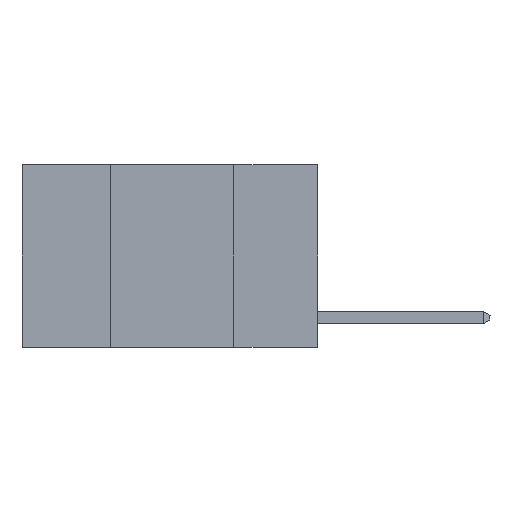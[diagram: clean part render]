
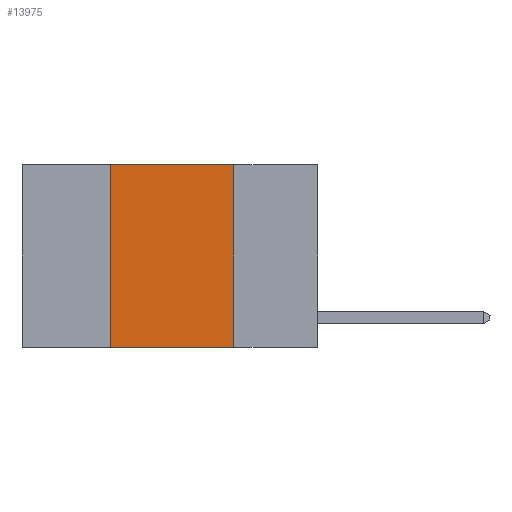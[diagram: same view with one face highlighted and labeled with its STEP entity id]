
A CAD part, left-side view. The second image highlights one B-rep face of the part: STEP entity #13975.
In plain terms, the highlighted planar face has unit normal (-1, 0, 0).
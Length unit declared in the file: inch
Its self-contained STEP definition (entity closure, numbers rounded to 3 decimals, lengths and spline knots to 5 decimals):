
#457 = CARTESIAN_POINT ( 'NONE',  ( 0., 0.6, 0. ) ) ;
#1369 = CARTESIAN_POINT ( 'NONE',  ( 0., 0.17, 0. ) ) ;
#2484 = VECTOR ( 'NONE', #20574, 39.37008 ) ;
#2641 = PLANE ( 'NONE',  #3850 ) ;
#2742 = EDGE_CURVE ( 'NONE', #21533, #28099, #12007, .T. ) ;
#2953 = VECTOR ( 'NONE', #18723, 39.37008 ) ;
#3850 = AXIS2_PLACEMENT_3D ( 'NONE', #457, #18011, #4877 ) ;
#4068 = CARTESIAN_POINT ( 'NONE',  ( 0., 0.17, 0. ) ) ;
#4877 = DIRECTION ( 'NONE',  ( 0., 0., -1. ) ) ;
#5718 = EDGE_CURVE ( 'NONE', #21533, #20551, #14908, .T. ) ;
#6151 = VECTOR ( 'NONE', #18054, 39.37008 ) ;
#6506 = ORIENTED_EDGE ( 'NONE', *, *, #10571, .F. ) ;
#7105 = CARTESIAN_POINT ( 'NONE',  ( 0., 0.17, -0.37 ) ) ;
#8156 = VECTOR ( 'NONE', #25834, 39.37008 ) ;
#8691 = CARTESIAN_POINT ( 'NONE',  ( 0., 0.42, -0.37 ) ) ;
#8816 = LINE ( 'NONE', #16555, #2953 ) ;
#10149 = EDGE_CURVE ( 'NONE', #21823, #28099, #19775, .T. ) ;
#10571 = EDGE_CURVE ( 'NONE', #20551, #21823, #8816, .T. ) ;
#11197 = ORIENTED_EDGE ( 'NONE', *, *, #5718, .F. ) ;
#12007 = LINE ( 'NONE', #24416, #6151 ) ;
#13975 = ADVANCED_FACE ( 'NONE', ( #17517 ), #2641, .F. ) ;
#14908 = LINE ( 'NONE', #16275, #2484 ) ;
#16275 = CARTESIAN_POINT ( 'NONE',  ( 0., 0.42, 0. ) ) ;
#16555 = CARTESIAN_POINT ( 'NONE',  ( 0., 0.6, 0. ) ) ;
#17517 = FACE_OUTER_BOUND ( 'NONE', #19127, .T. ) ;
#18011 = DIRECTION ( 'NONE',  ( 1., 0., 0. ) ) ;
#18054 = DIRECTION ( 'NONE',  ( 0., -1., 0. ) ) ;
#18723 = DIRECTION ( 'NONE',  ( 0., -1., 0. ) ) ;
#19127 = EDGE_LOOP ( 'NONE', ( #27038, #6506, #11197, #19301 ) ) ;
#19301 = ORIENTED_EDGE ( 'NONE', *, *, #2742, .T. ) ;
#19775 = LINE ( 'NONE', #4068, #8156 ) ;
#20551 = VERTEX_POINT ( 'NONE', #27121 ) ;
#20574 = DIRECTION ( 'NONE',  ( 0., 0., 1. ) ) ;
#21533 = VERTEX_POINT ( 'NONE', #8691 ) ;
#21823 = VERTEX_POINT ( 'NONE', #1369 ) ;
#24416 = CARTESIAN_POINT ( 'NONE',  ( 0., 0.6, -0.37 ) ) ;
#25834 = DIRECTION ( 'NONE',  ( 0., 0., -1. ) ) ;
#27038 = ORIENTED_EDGE ( 'NONE', *, *, #10149, .F. ) ;
#27121 = CARTESIAN_POINT ( 'NONE',  ( 0., 0.42, 0. ) ) ;
#28099 = VERTEX_POINT ( 'NONE', #7105 ) ;
